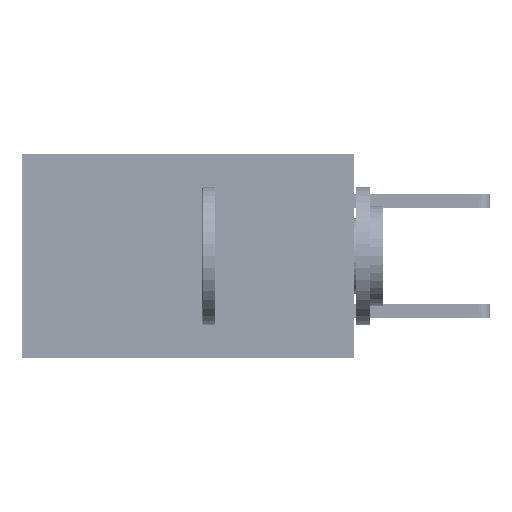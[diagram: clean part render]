
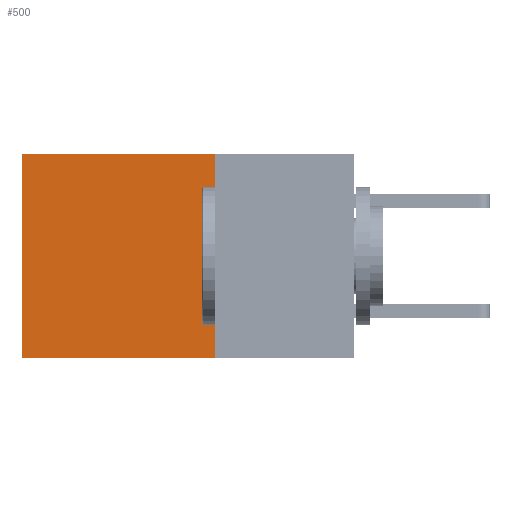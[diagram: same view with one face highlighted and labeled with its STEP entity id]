
A CAD part, left-side view. The second image highlights one B-rep face of the part: STEP entity #500.
In plain terms, the highlighted planar face has unit normal (-1, 0, 0).
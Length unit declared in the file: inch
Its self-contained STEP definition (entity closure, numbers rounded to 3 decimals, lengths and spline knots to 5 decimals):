
#500 = ADVANCED_FACE ( 'NONE', ( #41703 ), #45200, .F. ) ;
#952 = ORIENTED_EDGE ( 'NONE', *, *, #18845, .F. ) ;
#2866 = ORIENTED_EDGE ( 'NONE', *, *, #45644, .T. ) ;
#6269 = ORIENTED_EDGE ( 'NONE', *, *, #22781, .T. ) ;
#6532 = DIRECTION ( 'NONE',  ( 0., 0., -1. ) ) ;
#6899 = CARTESIAN_POINT ( 'NONE',  ( 0.2875, 0.25, 0. ) ) ;
#7097 = VECTOR ( 'NONE', #15115, 39.37008 ) ;
#7101 = DIRECTION ( 'NONE',  ( 0., 0., -1. ) ) ;
#7955 = AXIS2_PLACEMENT_3D ( 'NONE', #22558, #18563, #7101 ) ;
#8122 = VERTEX_POINT ( 'NONE', #20679 ) ;
#9820 = LINE ( 'NONE', #40459, #46657 ) ;
#10156 = EDGE_LOOP ( 'NONE', ( #2866, #34728, #952, #6269 ) ) ;
#12024 = EDGE_CURVE ( 'NONE', #8122, #37025, #9820, .T. ) ;
#14167 = VECTOR ( 'NONE', #36028, 39.37008 ) ;
#14375 = LINE ( 'NONE', #6899, #7097 ) ;
#15115 = DIRECTION ( 'NONE',  ( 0., 1., 0. ) ) ;
#15530 = VERTEX_POINT ( 'NONE', #45209 ) ;
#18563 = DIRECTION ( 'NONE',  ( 1., 0., 0. ) ) ;
#18845 = EDGE_CURVE ( 'NONE', #42354, #8122, #21522, .T. ) ;
#20679 = CARTESIAN_POINT ( 'NONE',  ( 0.2875, 0.25, -0.37 ) ) ;
#21522 = LINE ( 'NONE', #43911, #35597 ) ;
#21542 = DIRECTION ( 'NONE',  ( 0., 1., 0. ) ) ;
#22558 = CARTESIAN_POINT ( 'NONE',  ( 0.2875, 0.25, 0. ) ) ;
#22781 = EDGE_CURVE ( 'NONE', #42354, #15530, #14375, .T. ) ;
#26888 = CARTESIAN_POINT ( 'NONE',  ( 0.2875, 0.6, -0.37 ) ) ;
#28317 = CARTESIAN_POINT ( 'NONE',  ( 0.2875, 0.6, 0. ) ) ;
#34728 = ORIENTED_EDGE ( 'NONE', *, *, #12024, .F. ) ;
#35292 = LINE ( 'NONE', #28317, #14167 ) ;
#35597 = VECTOR ( 'NONE', #6532, 39.37008 ) ;
#36028 = DIRECTION ( 'NONE',  ( 0., 0., -1. ) ) ;
#37025 = VERTEX_POINT ( 'NONE', #26888 ) ;
#40459 = CARTESIAN_POINT ( 'NONE',  ( 0.2875, 0.25, -0.37 ) ) ;
#41703 = FACE_OUTER_BOUND ( 'NONE', #10156, .T. ) ;
#42354 = VERTEX_POINT ( 'NONE', #48791 ) ;
#43911 = CARTESIAN_POINT ( 'NONE',  ( 0.2875, 0.25, 0. ) ) ;
#45200 = PLANE ( 'NONE',  #7955 ) ;
#45209 = CARTESIAN_POINT ( 'NONE',  ( 0.2875, 0.6, 0. ) ) ;
#45644 = EDGE_CURVE ( 'NONE', #15530, #37025, #35292, .T. ) ;
#46657 = VECTOR ( 'NONE', #21542, 39.37008 ) ;
#48791 = CARTESIAN_POINT ( 'NONE',  ( 0.2875, 0.25, 0. ) ) ;
